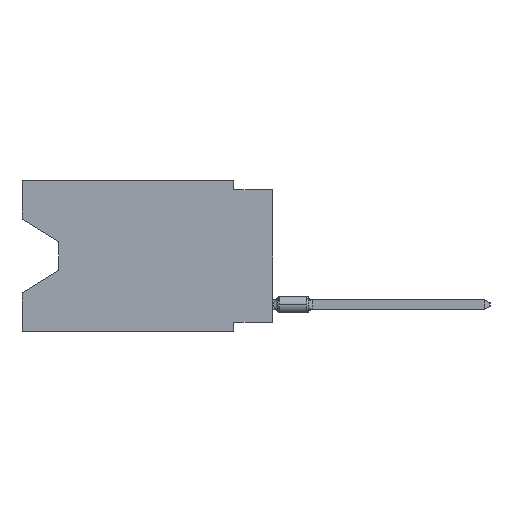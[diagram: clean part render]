
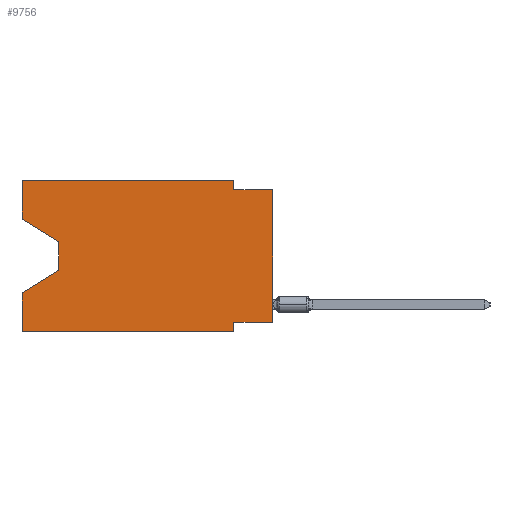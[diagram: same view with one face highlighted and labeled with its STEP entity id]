
A CAD part, left-side view. The second image highlights one B-rep face of the part: STEP entity #9756.
In plain terms, the highlighted planar face has unit normal (-1, 0, 0).
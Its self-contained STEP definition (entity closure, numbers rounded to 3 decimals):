
#799 = DIRECTION ( 'NONE',  ( 0., -0.855, -0.519 ) ) ;
#1015 = VECTOR ( 'NONE', #14441, 1000. ) ;
#1148 = VECTOR ( 'NONE', #12206, 1000. ) ;
#3059 = CARTESIAN_POINT ( 'NONE',  ( 0., 13.97, -5.893 ) ) ;
#4471 = CARTESIAN_POINT ( 'NONE',  ( 0., 0., -9.271 ) ) ;
#4685 = CARTESIAN_POINT ( 'NONE',  ( 0., 2.54, -9.906 ) ) ;
#5104 = LINE ( 'NONE', #4685, #36468 ) ;
#5346 = CARTESIAN_POINT ( 'NONE',  ( 0., 16.383, 0. ) ) ;
#5441 = ORIENTED_EDGE ( 'NONE', *, *, #13212, .T. ) ;
#5892 = CARTESIAN_POINT ( 'NONE',  ( 0., 0., -0.635 ) ) ;
#6013 = VERTEX_POINT ( 'NONE', #17734 ) ;
#6861 = VECTOR ( 'NONE', #34354, 1000. ) ;
#7448 = LINE ( 'NONE', #38356, #7501 ) ;
#7501 = VECTOR ( 'NONE', #35304, 1000. ) ;
#8412 = FACE_OUTER_BOUND ( 'NONE', #12954, .T. ) ;
#8752 = EDGE_CURVE ( 'NONE', #15702, #17906, #33310, .T. ) ;
#8848 = CARTESIAN_POINT ( 'NONE',  ( 0., 0., -0.635 ) ) ;
#9010 = ORIENTED_EDGE ( 'NONE', *, *, #19859, .T. ) ;
#9343 = LINE ( 'NONE', #24827, #6861 ) ;
#9469 = VECTOR ( 'NONE', #18293, 1000. ) ;
#9564 = CARTESIAN_POINT ( 'NONE',  ( 0., 16.383, -9.906 ) ) ;
#9661 = VERTEX_POINT ( 'NONE', #27150 ) ;
#9756 = ADVANCED_FACE ( 'NONE', ( #8412 ), #33220, .F. ) ;
#9910 = CARTESIAN_POINT ( 'NONE',  ( 0., 2.54, -9.906 ) ) ;
#10256 = VERTEX_POINT ( 'NONE', #13431 ) ;
#11361 = LINE ( 'NONE', #36347, #12086 ) ;
#11711 = LINE ( 'NONE', #8848, #27871 ) ;
#11977 = VERTEX_POINT ( 'NONE', #3059 ) ;
#12086 = VECTOR ( 'NONE', #17273, 1000. ) ;
#12206 = DIRECTION ( 'NONE',  ( 0., 0.855, -0.519 ) ) ;
#12523 = EDGE_CURVE ( 'NONE', #26863, #13813, #21760, .T. ) ;
#12615 = EDGE_CURVE ( 'NONE', #6013, #12960, #7448, .T. ) ;
#12912 = ORIENTED_EDGE ( 'NONE', *, *, #21093, .F. ) ;
#12954 = EDGE_LOOP ( 'NONE', ( #5441, #24243, #9010, #23109, #27283, #38024, #26950, #27639, #38457, #38816, #19266, #12912 ) ) ;
#12960 = VERTEX_POINT ( 'NONE', #21324 ) ;
#12961 = VECTOR ( 'NONE', #32615, 1000. ) ;
#13212 = EDGE_CURVE ( 'NONE', #9661, #21591, #37421, .T. ) ;
#13431 = CARTESIAN_POINT ( 'NONE',  ( 0., 2.54, -0.635 ) ) ;
#13813 = VERTEX_POINT ( 'NONE', #9910 ) ;
#14441 = DIRECTION ( 'NONE',  ( 0., 0., 1. ) ) ;
#14545 = CARTESIAN_POINT ( 'NONE',  ( 0., 2.54, -9.271 ) ) ;
#14559 = AXIS2_PLACEMENT_3D ( 'NONE', #5346, #29592, #17784 ) ;
#15702 = VERTEX_POINT ( 'NONE', #4471 ) ;
#15838 = EDGE_CURVE ( 'NONE', #26863, #28494, #26861, .T. ) ;
#16225 = CARTESIAN_POINT ( 'NONE',  ( 0., 16.383, -7.36 ) ) ;
#16741 = VECTOR ( 'NONE', #799, 1000. ) ;
#17273 = DIRECTION ( 'NONE',  ( 0., 0., -1. ) ) ;
#17734 = CARTESIAN_POINT ( 'NONE',  ( 0., 16.383, 0. ) ) ;
#17784 = DIRECTION ( 'NONE',  ( 0., 0., -1. ) ) ;
#17906 = VERTEX_POINT ( 'NONE', #14545 ) ;
#18293 = DIRECTION ( 'NONE',  ( 0., -1., 0. ) ) ;
#19266 = ORIENTED_EDGE ( 'NONE', *, *, #12615, .F. ) ;
#19859 = EDGE_CURVE ( 'NONE', #11977, #28494, #21575, .T. ) ;
#20430 = CARTESIAN_POINT ( 'NONE',  ( 0., 13.97, -4.013 ) ) ;
#20681 = DIRECTION ( 'NONE',  ( 0., -1., 0. ) ) ;
#21093 = EDGE_CURVE ( 'NONE', #9661, #6013, #9343, .T. ) ;
#21324 = CARTESIAN_POINT ( 'NONE',  ( 0., 2.54, 0. ) ) ;
#21575 = LINE ( 'NONE', #25224, #1148 ) ;
#21591 = VERTEX_POINT ( 'NONE', #24188 ) ;
#21760 = LINE ( 'NONE', #28056, #9469 ) ;
#22947 = CARTESIAN_POINT ( 'NONE',  ( 0., 0., 0. ) ) ;
#23109 = ORIENTED_EDGE ( 'NONE', *, *, #15838, .F. ) ;
#24188 = CARTESIAN_POINT ( 'NONE',  ( 0., 13.97, -4.013 ) ) ;
#24243 = ORIENTED_EDGE ( 'NONE', *, *, #26223, .T. ) ;
#24827 = CARTESIAN_POINT ( 'NONE',  ( 0., 16.383, 0. ) ) ;
#25224 = CARTESIAN_POINT ( 'NONE',  ( 0., 13.97, -5.893 ) ) ;
#25791 = LINE ( 'NONE', #22947, #33484 ) ;
#25841 = EDGE_CURVE ( 'NONE', #10256, #28018, #11711, .T. ) ;
#26223 = EDGE_CURVE ( 'NONE', #21591, #11977, #38890, .T. ) ;
#26861 = LINE ( 'NONE', #33940, #1015 ) ;
#26863 = VERTEX_POINT ( 'NONE', #9564 ) ;
#26884 = DIRECTION ( 'NONE',  ( 0., 0., -1. ) ) ;
#26950 = ORIENTED_EDGE ( 'NONE', *, *, #8752, .F. ) ;
#27035 = DIRECTION ( 'NONE',  ( 0., 1., 0. ) ) ;
#27150 = CARTESIAN_POINT ( 'NONE',  ( 0., 16.383, -2.546 ) ) ;
#27283 = ORIENTED_EDGE ( 'NONE', *, *, #12523, .T. ) ;
#27639 = ORIENTED_EDGE ( 'NONE', *, *, #37249, .T. ) ;
#27871 = VECTOR ( 'NONE', #20681, 1000. ) ;
#28018 = VERTEX_POINT ( 'NONE', #5892 ) ;
#28056 = CARTESIAN_POINT ( 'NONE',  ( 0., 16.383, -9.906 ) ) ;
#28494 = VERTEX_POINT ( 'NONE', #16225 ) ;
#29450 = VECTOR ( 'NONE', #27035, 1000. ) ;
#29592 = DIRECTION ( 'NONE',  ( 1., 0., 0. ) ) ;
#30628 = EDGE_CURVE ( 'NONE', #17906, #13813, #5104, .T. ) ;
#30694 = CARTESIAN_POINT ( 'NONE',  ( 0., 0., -9.271 ) ) ;
#32615 = DIRECTION ( 'NONE',  ( 0., 0., -1. ) ) ;
#33220 = PLANE ( 'NONE',  #14559 ) ;
#33310 = LINE ( 'NONE', #30694, #29450 ) ;
#33484 = VECTOR ( 'NONE', #38148, 1000. ) ;
#33940 = CARTESIAN_POINT ( 'NONE',  ( 0., 16.383, 0. ) ) ;
#34354 = DIRECTION ( 'NONE',  ( 0., 0., 1. ) ) ;
#35304 = DIRECTION ( 'NONE',  ( 0., -1., 0. ) ) ;
#36347 = CARTESIAN_POINT ( 'NONE',  ( 0., 2.54, 0. ) ) ;
#36468 = VECTOR ( 'NONE', #26884, 1000. ) ;
#36973 = EDGE_CURVE ( 'NONE', #12960, #10256, #11361, .T. ) ;
#37216 = CARTESIAN_POINT ( 'NONE',  ( 0., 16.383, -2.546 ) ) ;
#37249 = EDGE_CURVE ( 'NONE', #15702, #28018, #25791, .T. ) ;
#37421 = LINE ( 'NONE', #37216, #16741 ) ;
#38024 = ORIENTED_EDGE ( 'NONE', *, *, #30628, .F. ) ;
#38148 = DIRECTION ( 'NONE',  ( 0., 0., 1. ) ) ;
#38356 = CARTESIAN_POINT ( 'NONE',  ( 0., 16.383, 0. ) ) ;
#38457 = ORIENTED_EDGE ( 'NONE', *, *, #25841, .F. ) ;
#38816 = ORIENTED_EDGE ( 'NONE', *, *, #36973, .F. ) ;
#38890 = LINE ( 'NONE', #20430, #12961 ) ;
